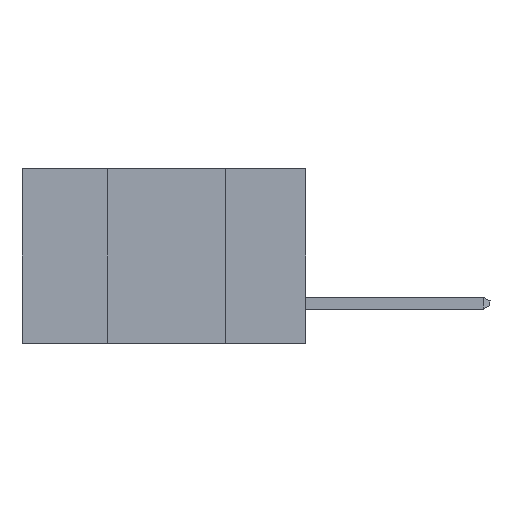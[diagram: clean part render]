
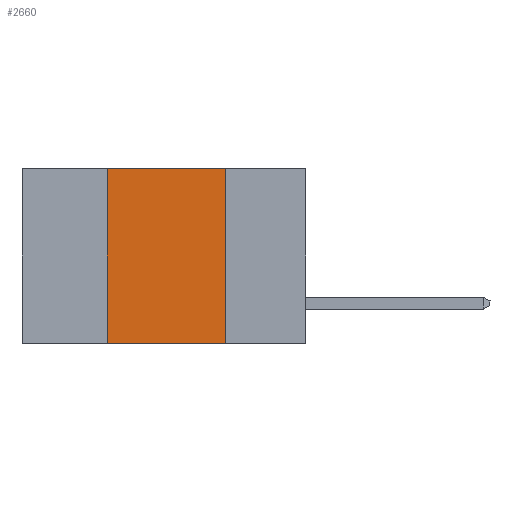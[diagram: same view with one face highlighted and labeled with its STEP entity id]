
A CAD part, left-side view. The second image highlights one B-rep face of the part: STEP entity #2660.
In plain terms, the highlighted planar face has unit normal (-1, 0, 0).
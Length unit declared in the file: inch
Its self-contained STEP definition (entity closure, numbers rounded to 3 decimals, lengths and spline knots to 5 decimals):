
#450 = AXIS2_PLACEMENT_3D ( 'NONE', #7287, #6988, #5109 ) ;
#706 = CARTESIAN_POINT ( 'NONE',  ( 0., 0.17, -0.37 ) ) ;
#1261 = CARTESIAN_POINT ( 'NONE',  ( 0., 0.42, -0.37 ) ) ;
#1826 = CARTESIAN_POINT ( 'NONE',  ( 0., 0.42, 0. ) ) ;
#2137 = DIRECTION ( 'NONE',  ( 0., -1., 0. ) ) ;
#2660 = ADVANCED_FACE ( 'NONE', ( #5985 ), #3868, .F. ) ;
#2856 = VECTOR ( 'NONE', #6288, 39.37008 ) ;
#3537 = CARTESIAN_POINT ( 'NONE',  ( 0., 0.17, -0.37 ) ) ;
#3582 = ORIENTED_EDGE ( 'NONE', *, *, #6739, .F. ) ;
#3868 = PLANE ( 'NONE',  #450 ) ;
#4411 = CARTESIAN_POINT ( 'NONE',  ( 0., 0.6, 0. ) ) ;
#5109 = DIRECTION ( 'NONE',  ( 0., 0., -1. ) ) ;
#5158 = EDGE_CURVE ( 'NONE', #12788, #5924, #14221, .T. ) ;
#5893 = ORIENTED_EDGE ( 'NONE', *, *, #6528, .T. ) ;
#5924 = VERTEX_POINT ( 'NONE', #10482 ) ;
#5975 = ORIENTED_EDGE ( 'NONE', *, *, #5158, .F. ) ;
#5985 = FACE_OUTER_BOUND ( 'NONE', #11684, .T. ) ;
#6288 = DIRECTION ( 'NONE',  ( 0., -1., 0. ) ) ;
#6528 = EDGE_CURVE ( 'NONE', #12164, #6546, #10653, .T. ) ;
#6546 = VERTEX_POINT ( 'NONE', #706 ) ;
#6739 = EDGE_CURVE ( 'NONE', #12164, #12788, #13559, .T. ) ;
#6976 = ORIENTED_EDGE ( 'NONE', *, *, #7613, .F. ) ;
#6988 = DIRECTION ( 'NONE',  ( 1., 0., 0. ) ) ;
#7096 = LINE ( 'NONE', #3537, #10648 ) ;
#7287 = CARTESIAN_POINT ( 'NONE',  ( 0., 0.6, 0. ) ) ;
#7613 = EDGE_CURVE ( 'NONE', #5924, #6546, #7096, .T. ) ;
#7975 = CARTESIAN_POINT ( 'NONE',  ( 0., 0.42, -0.37 ) ) ;
#8180 = DIRECTION ( 'NONE',  ( 0., 0., -1. ) ) ;
#10482 = CARTESIAN_POINT ( 'NONE',  ( 0., 0.17, 0. ) ) ;
#10648 = VECTOR ( 'NONE', #8180, 39.37008 ) ;
#10653 = LINE ( 'NONE', #11643, #2856 ) ;
#11643 = CARTESIAN_POINT ( 'NONE',  ( 0., 0.6, -0.37 ) ) ;
#11684 = EDGE_LOOP ( 'NONE', ( #6976, #5975, #3582, #5893 ) ) ;
#12164 = VERTEX_POINT ( 'NONE', #7975 ) ;
#12346 = DIRECTION ( 'NONE',  ( 0., 0., 1. ) ) ;
#12788 = VERTEX_POINT ( 'NONE', #1826 ) ;
#13308 = VECTOR ( 'NONE', #12346, 39.37008 ) ;
#13559 = LINE ( 'NONE', #1261, #13308 ) ;
#13887 = VECTOR ( 'NONE', #2137, 39.37008 ) ;
#14221 = LINE ( 'NONE', #4411, #13887 ) ;
